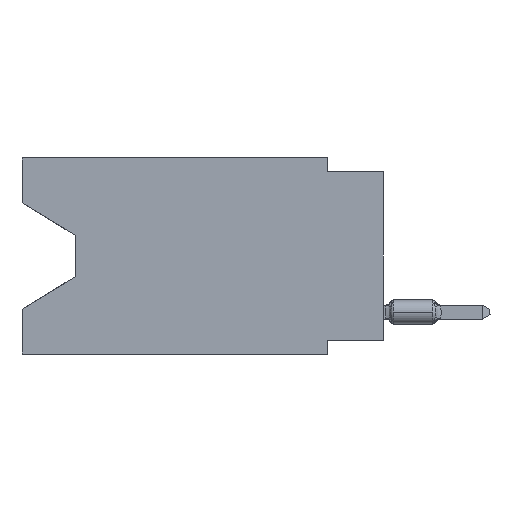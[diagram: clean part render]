
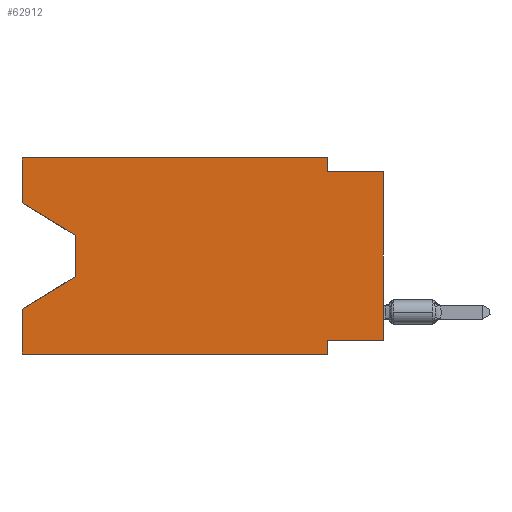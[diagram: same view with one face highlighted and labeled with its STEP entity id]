
A CAD part, left-side view. The second image highlights one B-rep face of the part: STEP entity #62912.
In plain terms, the highlighted planar face has unit normal (-1, 0, 0).
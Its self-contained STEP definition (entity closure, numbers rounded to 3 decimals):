
#742 = CARTESIAN_POINT ( 'NONE',  ( 0., 0., -0.635 ) ) ;
#791 = DIRECTION ( 'NONE',  ( 0., 0., -1. ) ) ;
#1134 = CARTESIAN_POINT ( 'NONE',  ( 0., 16.383, -8.89 ) ) ;
#2475 = CARTESIAN_POINT ( 'NONE',  ( 0., 16.383, -2.038 ) ) ;
#3364 = VERTEX_POINT ( 'NONE', #4281 ) ;
#3439 = LINE ( 'NONE', #23433, #57014 ) ;
#3965 = VECTOR ( 'NONE', #59883, 1000. ) ;
#4254 = EDGE_CURVE ( 'NONE', #48647, #32078, #3439, .T. ) ;
#4281 = CARTESIAN_POINT ( 'NONE',  ( 0., 2.54, -0.635 ) ) ;
#4948 = VERTEX_POINT ( 'NONE', #26260 ) ;
#5186 = VERTEX_POINT ( 'NONE', #42622 ) ;
#5441 = DIRECTION ( 'NONE',  ( 0., 0., -1. ) ) ;
#5844 = CARTESIAN_POINT ( 'NONE',  ( 0., 16.383, 0. ) ) ;
#6711 = VECTOR ( 'NONE', #48763, 1000. ) ;
#10249 = LINE ( 'NONE', #742, #18823 ) ;
#10451 = VECTOR ( 'NONE', #17542, 1000. ) ;
#10767 = CARTESIAN_POINT ( 'NONE',  ( 0., 16.383, 0. ) ) ;
#12687 = VERTEX_POINT ( 'NONE', #39319 ) ;
#13342 = ORIENTED_EDGE ( 'NONE', *, *, #17450, .F. ) ;
#13349 = LINE ( 'NONE', #27461, #6711 ) ;
#13622 = ORIENTED_EDGE ( 'NONE', *, *, #39190, .T. ) ;
#14537 = DIRECTION ( 'NONE',  ( 0., 0., -1. ) ) ;
#15575 = VERTEX_POINT ( 'NONE', #46505 ) ;
#17450 = EDGE_CURVE ( 'NONE', #15575, #32078, #50762, .T. ) ;
#17542 = DIRECTION ( 'NONE',  ( 0., -0.855, -0.519 ) ) ;
#17725 = ORIENTED_EDGE ( 'NONE', *, *, #28591, .F. ) ;
#17948 = CARTESIAN_POINT ( 'NONE',  ( 0., 2.54, -8.89 ) ) ;
#18017 = CARTESIAN_POINT ( 'NONE',  ( 0., 0., -8.255 ) ) ;
#18823 = VECTOR ( 'NONE', #25321, 1000. ) ;
#18892 = EDGE_CURVE ( 'NONE', #34217, #48793, #40203, .T. ) ;
#19476 = DIRECTION ( 'NONE',  ( 0., 0.855, -0.519 ) ) ;
#19769 = CARTESIAN_POINT ( 'NONE',  ( 0., 2.54, 0. ) ) ;
#21484 = EDGE_CURVE ( 'NONE', #4948, #3364, #49290, .T. ) ;
#21497 = DIRECTION ( 'NONE',  ( 0., 0., 1. ) ) ;
#21968 = ORIENTED_EDGE ( 'NONE', *, *, #21484, .F. ) ;
#23433 = CARTESIAN_POINT ( 'NONE',  ( 0., 13.97, -5.385 ) ) ;
#23951 = EDGE_CURVE ( 'NONE', #12687, #48647, #45429, .T. ) ;
#25321 = DIRECTION ( 'NONE',  ( 0., -1., 0. ) ) ;
#25433 = LINE ( 'NONE', #36257, #52328 ) ;
#25730 = ORIENTED_EDGE ( 'NONE', *, *, #62256, .F. ) ;
#26008 = CARTESIAN_POINT ( 'NONE',  ( 0., 0., -0.635 ) ) ;
#26011 = DIRECTION ( 'NONE',  ( 1., 0., 0. ) ) ;
#26260 = CARTESIAN_POINT ( 'NONE',  ( 0., 2.54, 0. ) ) ;
#26397 = VERTEX_POINT ( 'NONE', #10767 ) ;
#26674 = PLANE ( 'NONE',  #63288 ) ;
#27388 = ORIENTED_EDGE ( 'NONE', *, *, #18892, .T. ) ;
#27461 = CARTESIAN_POINT ( 'NONE',  ( 0., 16.383, 0. ) ) ;
#28591 = EDGE_CURVE ( 'NONE', #34217, #5186, #62932, .T. ) ;
#29698 = CARTESIAN_POINT ( 'NONE',  ( 0., 16.383, -2.038 ) ) ;
#32078 = VERTEX_POINT ( 'NONE', #52191 ) ;
#32589 = VERTEX_POINT ( 'NONE', #29698 ) ;
#32944 = LINE ( 'NONE', #2475, #10451 ) ;
#34217 = VERTEX_POINT ( 'NONE', #39689 ) ;
#34891 = CARTESIAN_POINT ( 'NONE',  ( 0., 13.97, -5.385 ) ) ;
#35588 = ORIENTED_EDGE ( 'NONE', *, *, #59234, .F. ) ;
#35758 = EDGE_LOOP ( 'NONE', ( #58822, #43368, #59343, #13342, #13622, #49442, #17725, #27388, #35588, #21968, #25730, #40571 ) ) ;
#36144 = LINE ( 'NONE', #46304, #57536 ) ;
#36257 = CARTESIAN_POINT ( 'NONE',  ( 0., 16.383, 0. ) ) ;
#37573 = VECTOR ( 'NONE', #14537, 1000. ) ;
#39190 = EDGE_CURVE ( 'NONE', #15575, #52076, #40139, .T. ) ;
#39319 = CARTESIAN_POINT ( 'NONE',  ( 0., 13.97, -3.505 ) ) ;
#39689 = CARTESIAN_POINT ( 'NONE',  ( 0., 0., -8.255 ) ) ;
#40139 = LINE ( 'NONE', #1134, #56890 ) ;
#40203 = LINE ( 'NONE', #64483, #3965 ) ;
#40571 = ORIENTED_EDGE ( 'NONE', *, *, #61416, .F. ) ;
#42622 = CARTESIAN_POINT ( 'NONE',  ( 0., 2.54, -8.255 ) ) ;
#43099 = DIRECTION ( 'NONE',  ( 0., 0., 1. ) ) ;
#43368 = ORIENTED_EDGE ( 'NONE', *, *, #23951, .T. ) ;
#45429 = LINE ( 'NONE', #45754, #51012 ) ;
#45709 = DIRECTION ( 'NONE',  ( 0., -1., 0. ) ) ;
#45754 = CARTESIAN_POINT ( 'NONE',  ( 0., 13.97, -3.505 ) ) ;
#46304 = CARTESIAN_POINT ( 'NONE',  ( 0., 2.54, -8.89 ) ) ;
#46505 = CARTESIAN_POINT ( 'NONE',  ( 0., 16.383, -8.89 ) ) ;
#48647 = VERTEX_POINT ( 'NONE', #34891 ) ;
#48763 = DIRECTION ( 'NONE',  ( 0., -1., 0. ) ) ;
#48793 = VERTEX_POINT ( 'NONE', #26008 ) ;
#49290 = LINE ( 'NONE', #19769, #37573 ) ;
#49442 = ORIENTED_EDGE ( 'NONE', *, *, #59279, .F. ) ;
#50270 = VECTOR ( 'NONE', #58018, 1000. ) ;
#50762 = LINE ( 'NONE', #5844, #58940 ) ;
#51012 = VECTOR ( 'NONE', #5441, 1000. ) ;
#51216 = DIRECTION ( 'NONE',  ( 0., 0., -1. ) ) ;
#52076 = VERTEX_POINT ( 'NONE', #17948 ) ;
#52191 = CARTESIAN_POINT ( 'NONE',  ( 0., 16.383, -6.852 ) ) ;
#52328 = VECTOR ( 'NONE', #21497, 1000. ) ;
#56890 = VECTOR ( 'NONE', #45709, 1000. ) ;
#57014 = VECTOR ( 'NONE', #19476, 1000. ) ;
#57536 = VECTOR ( 'NONE', #51216, 1000. ) ;
#58018 = DIRECTION ( 'NONE',  ( 0., 1., 0. ) ) ;
#58822 = ORIENTED_EDGE ( 'NONE', *, *, #61475, .T. ) ;
#58940 = VECTOR ( 'NONE', #43099, 1000. ) ;
#59234 = EDGE_CURVE ( 'NONE', #3364, #48793, #10249, .T. ) ;
#59279 = EDGE_CURVE ( 'NONE', #5186, #52076, #36144, .T. ) ;
#59343 = ORIENTED_EDGE ( 'NONE', *, *, #4254, .T. ) ;
#59883 = DIRECTION ( 'NONE',  ( 0., 0., 1. ) ) ;
#60455 = FACE_OUTER_BOUND ( 'NONE', #35758, .T. ) ;
#61108 = CARTESIAN_POINT ( 'NONE',  ( 0., 16.383, 0. ) ) ;
#61416 = EDGE_CURVE ( 'NONE', #32589, #26397, #25433, .T. ) ;
#61475 = EDGE_CURVE ( 'NONE', #32589, #12687, #32944, .T. ) ;
#62256 = EDGE_CURVE ( 'NONE', #26397, #4948, #13349, .T. ) ;
#62912 = ADVANCED_FACE ( 'NONE', ( #60455 ), #26674, .F. ) ;
#62932 = LINE ( 'NONE', #18017, #50270 ) ;
#63288 = AXIS2_PLACEMENT_3D ( 'NONE', #61108, #26011, #791 ) ;
#64483 = CARTESIAN_POINT ( 'NONE',  ( 0., 0., 0. ) ) ;
